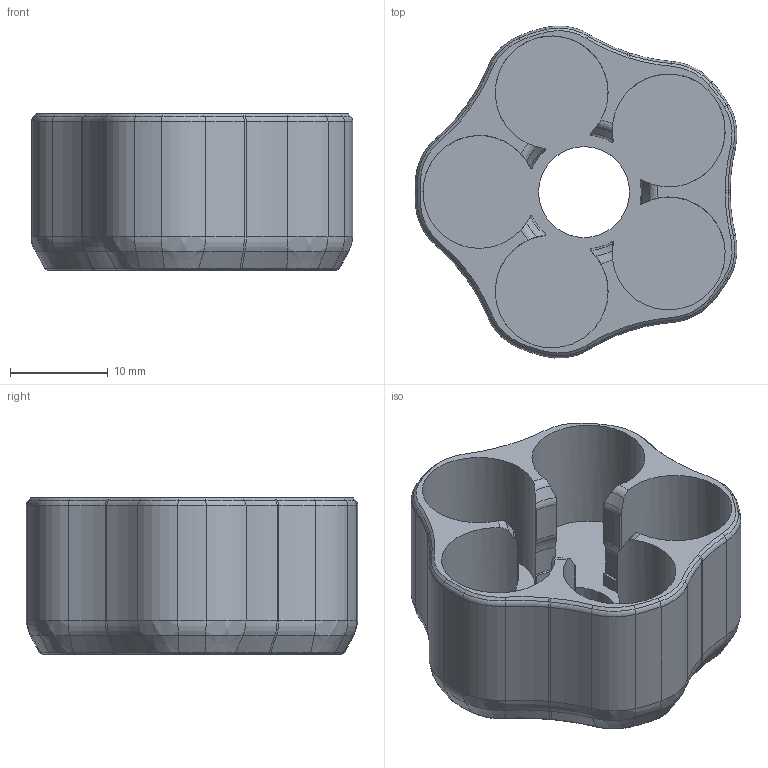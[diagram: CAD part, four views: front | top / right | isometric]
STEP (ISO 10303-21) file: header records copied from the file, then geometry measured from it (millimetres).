
FILE_DESCRIPTION(/* description */ (''),/* implementation_level */ '2;1');
FILE_NAME(/* name */ 'Cartridge Holder.step',/* time_stamp */ '2021-05-12T04:47:22-04:00',/* author */ (''),/* organization */ (''),/* preprocessor_version */ 'ST-DEVELOPER v18.1',/* originating_system */ 'Autodesk Translation Framework v10.6.0.1341',/* authorisation */ '');
FILE_SCHEMA (('AUTOMOTIVE_DESIGN { 1 0 10303 214 3 1 1 }'));
Length unit declared in the file: millimetre
Products named in the file (1): Cartridge Holder
Bounding box: 32.9 x 33.93 x 16 mm (x, y, z)
Volume: 5256.9 mm3; surface area: 5233.3 mm2
Topology: 1 solids, 1 shells, 268 faces, 634 edges, 370 vertices
Faces by surface type: cylinder 84, torus 83, cone 60, plane 26, bspline 15
Full cylindrical faces by diameter (mm): 9.3 x1
Entity records: 8126 total; most frequent: CARTESIAN_POINT 1853, DIRECTION 1444, ORIENTED_EDGE 1268, EDGE_CURVE 634, AXIS2_PLACEMENT_3D 630, CIRCLE 376, VERTEX_POINT 370, EDGE_LOOP 272
